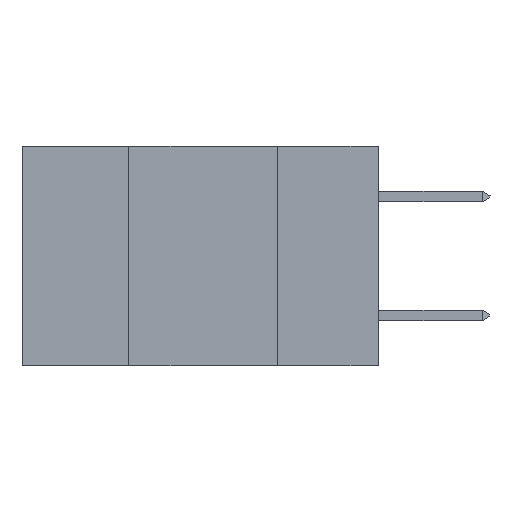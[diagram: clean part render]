
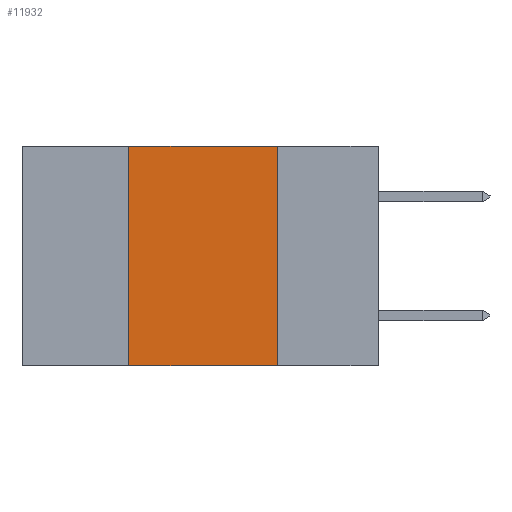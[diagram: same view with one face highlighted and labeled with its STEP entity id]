
A CAD part, left-side view. The second image highlights one B-rep face of the part: STEP entity #11932.
In plain terms, the highlighted planar face has unit normal (-1, 0, 0).
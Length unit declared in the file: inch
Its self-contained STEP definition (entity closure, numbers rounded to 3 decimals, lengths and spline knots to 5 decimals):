
#79 = DIRECTION ( 'NONE',  ( 0., 0., -1. ) ) ;
#158 = EDGE_LOOP ( 'NONE', ( #5061, #2566, #11911, #3853 ) ) ;
#242 = VECTOR ( 'NONE', #4803, 39.37008 ) ;
#352 = DIRECTION ( 'NONE',  ( 1., 0., 0. ) ) ;
#739 = LINE ( 'NONE', #6793, #12206 ) ;
#1625 = VECTOR ( 'NONE', #5915, 39.37008 ) ;
#1779 = EDGE_CURVE ( 'NONE', #1916, #5446, #7073, .T. ) ;
#1855 = VERTEX_POINT ( 'NONE', #8984 ) ;
#1916 = VERTEX_POINT ( 'NONE', #13048 ) ;
#2566 = ORIENTED_EDGE ( 'NONE', *, *, #1779, .F. ) ;
#3137 = PLANE ( 'NONE',  #7395 ) ;
#3537 = CARTESIAN_POINT ( 'NONE',  ( 0., 0.17, 0. ) ) ;
#3658 = VERTEX_POINT ( 'NONE', #5925 ) ;
#3718 = DIRECTION ( 'NONE',  ( 0., 0., 1. ) ) ;
#3853 = ORIENTED_EDGE ( 'NONE', *, *, #6176, .T. ) ;
#4043 = CARTESIAN_POINT ( 'NONE',  ( 0., 0.6, -0.37 ) ) ;
#4803 = DIRECTION ( 'NONE',  ( 0., -1., 0. ) ) ;
#4985 = LINE ( 'NONE', #9017, #1625 ) ;
#5009 = CARTESIAN_POINT ( 'NONE',  ( 0., 0.6, 0. ) ) ;
#5061 = ORIENTED_EDGE ( 'NONE', *, *, #10987, .F. ) ;
#5446 = VERTEX_POINT ( 'NONE', #3537 ) ;
#5915 = DIRECTION ( 'NONE',  ( 0., 0., -1. ) ) ;
#5925 = CARTESIAN_POINT ( 'NONE',  ( 0., 0.42, -0.37 ) ) ;
#6176 = EDGE_CURVE ( 'NONE', #3658, #1855, #7418, .T. ) ;
#6793 = CARTESIAN_POINT ( 'NONE',  ( 0., 0.42, -0.37 ) ) ;
#7073 = LINE ( 'NONE', #5009, #242 ) ;
#7395 = AXIS2_PLACEMENT_3D ( 'NONE', #11394, #352, #79 ) ;
#7418 = LINE ( 'NONE', #4043, #10444 ) ;
#8081 = DIRECTION ( 'NONE',  ( 0., -1., 0. ) ) ;
#8173 = FACE_OUTER_BOUND ( 'NONE', #158, .T. ) ;
#8984 = CARTESIAN_POINT ( 'NONE',  ( 0., 0.17, -0.37 ) ) ;
#9017 = CARTESIAN_POINT ( 'NONE',  ( 0., 0.17, -0.37 ) ) ;
#10444 = VECTOR ( 'NONE', #8081, 39.37008 ) ;
#10987 = EDGE_CURVE ( 'NONE', #5446, #1855, #4985, .T. ) ;
#11069 = EDGE_CURVE ( 'NONE', #3658, #1916, #739, .T. ) ;
#11394 = CARTESIAN_POINT ( 'NONE',  ( 0., 0.6, 0. ) ) ;
#11911 = ORIENTED_EDGE ( 'NONE', *, *, #11069, .F. ) ;
#11932 = ADVANCED_FACE ( 'NONE', ( #8173 ), #3137, .F. ) ;
#12206 = VECTOR ( 'NONE', #3718, 39.37008 ) ;
#13048 = CARTESIAN_POINT ( 'NONE',  ( 0., 0.42, 0. ) ) ;
